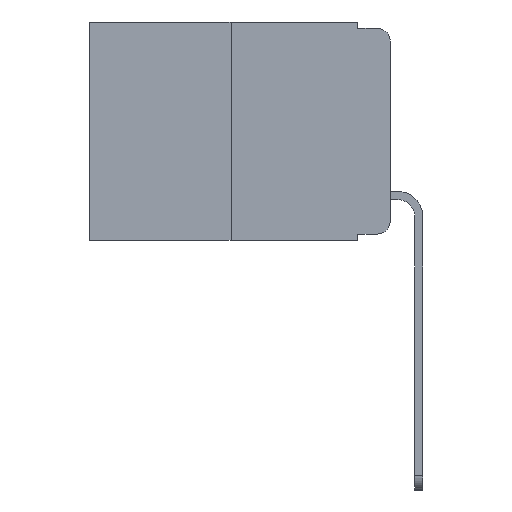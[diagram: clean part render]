
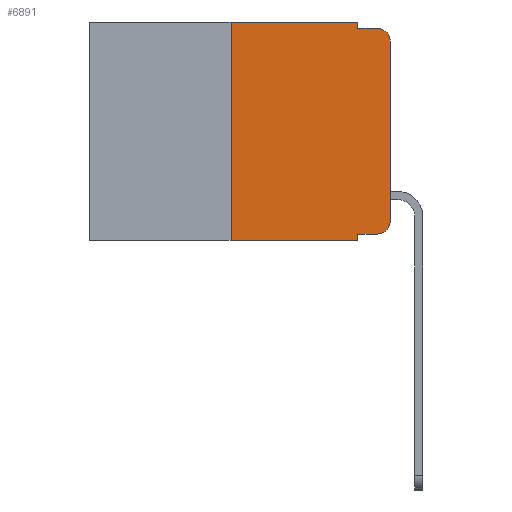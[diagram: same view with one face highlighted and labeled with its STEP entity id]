
A CAD part, left-side view. The second image highlights one B-rep face of the part: STEP entity #6891.
In plain terms, the highlighted planar face has unit normal (-1, 0, 0).
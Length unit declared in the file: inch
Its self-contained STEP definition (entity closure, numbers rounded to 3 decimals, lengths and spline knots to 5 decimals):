
#18 = ORIENTED_EDGE ( 'NONE', *, *, #57, .F. ) ;
#43 = CARTESIAN_POINT ( 'NONE',  ( 0., 0., 0. ) ) ;
#57 = EDGE_CURVE ( 'NONE', #5932, #10891, #1332, .T. ) ;
#103 = VERTEX_POINT ( 'NONE', #6061 ) ;
#205 = AXIS2_PLACEMENT_3D ( 'NONE', #3774, #10359, #4738 ) ;
#323 = ORIENTED_EDGE ( 'NONE', *, *, #4241, .F. ) ;
#609 = CARTESIAN_POINT ( 'NONE',  ( 0., 0.02, -0.333 ) ) ;
#680 = DIRECTION ( 'NONE',  ( 1., 0., 0. ) ) ;
#1033 = ORIENTED_EDGE ( 'NONE', *, *, #2720, .F. ) ;
#1242 = CARTESIAN_POINT ( 'NONE',  ( 0., 0.25, 0. ) ) ;
#1308 = ORIENTED_EDGE ( 'NONE', *, *, #7419, .T. ) ;
#1332 = LINE ( 'NONE', #3484, #6007 ) ;
#1449 = DIRECTION ( 'NONE',  ( 0., -1., 0. ) ) ;
#1610 = CARTESIAN_POINT ( 'NONE',  ( 0., 0., -0.03 ) ) ;
#1893 = ORIENTED_EDGE ( 'NONE', *, *, #2748, .T. ) ;
#1938 = DIRECTION ( 'NONE',  ( 0., -1., 0. ) ) ;
#2084 = DIRECTION ( 'NONE',  ( 0., 0., -1. ) ) ;
#2150 = ORIENTED_EDGE ( 'NONE', *, *, #2764, .F. ) ;
#2442 = VERTEX_POINT ( 'NONE', #1610 ) ;
#2446 = CARTESIAN_POINT ( 'NONE',  ( 0., 0.473, -0.343 ) ) ;
#2636 = ORIENTED_EDGE ( 'NONE', *, *, #9482, .T. ) ;
#2720 = EDGE_CURVE ( 'NONE', #10809, #6787, #6784, .T. ) ;
#2748 = EDGE_CURVE ( 'NONE', #2442, #6787, #11028, .T. ) ;
#2764 = EDGE_CURVE ( 'NONE', #10671, #10809, #3883, .T. ) ;
#2803 = EDGE_CURVE ( 'NONE', #3723, #2442, #7843, .T. ) ;
#3084 = CIRCLE ( 'NONE', #205, 0.02 ) ;
#3091 = CARTESIAN_POINT ( 'NONE',  ( 0., 0.051, 0. ) ) ;
#3484 = CARTESIAN_POINT ( 'NONE',  ( 0., 0.25, 0. ) ) ;
#3723 = VERTEX_POINT ( 'NONE', #11945 ) ;
#3735 = ORIENTED_EDGE ( 'NONE', *, *, #8161, .F. ) ;
#3774 = CARTESIAN_POINT ( 'NONE',  ( 0., 0.02, -0.313 ) ) ;
#3883 = LINE ( 'NONE', #3091, #6157 ) ;
#4241 = EDGE_CURVE ( 'NONE', #10979, #103, #8240, .T. ) ;
#4738 = DIRECTION ( 'NONE',  ( 0., 0., -1. ) ) ;
#4887 = CARTESIAN_POINT ( 'NONE',  ( 0., 0.473, 0. ) ) ;
#5195 = FACE_OUTER_BOUND ( 'NONE', #5410, .T. ) ;
#5410 = EDGE_LOOP ( 'NONE', ( #10068, #1893, #1033, #2150, #3735, #18, #2636, #323, #1308, #9926 ) ) ;
#5591 = VECTOR ( 'NONE', #1449, 39.37008 ) ;
#5630 = VECTOR ( 'NONE', #7836, 39.37008 ) ;
#5920 = LINE ( 'NONE', #2446, #5591 ) ;
#5932 = VERTEX_POINT ( 'NONE', #8410 ) ;
#5979 = DIRECTION ( 'NONE',  ( 0., 0., -1. ) ) ;
#6007 = VECTOR ( 'NONE', #7228, 39.37008 ) ;
#6061 = CARTESIAN_POINT ( 'NONE',  ( 0., 0.051, -0.343 ) ) ;
#6157 = VECTOR ( 'NONE', #2084, 39.37008 ) ;
#6293 = CARTESIAN_POINT ( 'NONE',  ( 0., 0.051, -0.333 ) ) ;
#6436 = LINE ( 'NONE', #10551, #11000 ) ;
#6784 = LINE ( 'NONE', #7641, #8996 ) ;
#6787 = VERTEX_POINT ( 'NONE', #9212 ) ;
#6821 = DIRECTION ( 'NONE',  ( 0., -1., 0. ) ) ;
#6888 = VECTOR ( 'NONE', #1938, 39.37008 ) ;
#6891 = ADVANCED_FACE ( 'NONE', ( #5195 ), #9555, .F. ) ;
#7151 = DIRECTION ( 'NONE',  ( 0., 0., 1. ) ) ;
#7228 = DIRECTION ( 'NONE',  ( 0., 0., 1. ) ) ;
#7317 = EDGE_CURVE ( 'NONE', #10431, #3723, #3084, .T. ) ;
#7419 = EDGE_CURVE ( 'NONE', #10979, #10431, #6436, .T. ) ;
#7641 = CARTESIAN_POINT ( 'NONE',  ( 0., 0.051, -0.01 ) ) ;
#7836 = DIRECTION ( 'NONE',  ( 0., 0., -1. ) ) ;
#7843 = LINE ( 'NONE', #43, #8126 ) ;
#8126 = VECTOR ( 'NONE', #7151, 39.37008 ) ;
#8161 = EDGE_CURVE ( 'NONE', #10891, #10671, #9364, .T. ) ;
#8240 = LINE ( 'NONE', #10496, #5630 ) ;
#8410 = CARTESIAN_POINT ( 'NONE',  ( 0., 0.25, -0.343 ) ) ;
#8667 = CARTESIAN_POINT ( 'NONE',  ( 0., 0.473, 0. ) ) ;
#8963 = CARTESIAN_POINT ( 'NONE',  ( 0., 0.051, -0.01 ) ) ;
#8996 = VECTOR ( 'NONE', #6821, 39.37008 ) ;
#9212 = CARTESIAN_POINT ( 'NONE',  ( 0., 0.02, -0.01 ) ) ;
#9364 = LINE ( 'NONE', #4887, #6888 ) ;
#9482 = EDGE_CURVE ( 'NONE', #5932, #103, #5920, .T. ) ;
#9555 = PLANE ( 'NONE',  #11297 ) ;
#9667 = DIRECTION ( 'NONE',  ( 0., -1., 0. ) ) ;
#9926 = ORIENTED_EDGE ( 'NONE', *, *, #7317, .T. ) ;
#10068 = ORIENTED_EDGE ( 'NONE', *, *, #2803, .T. ) ;
#10359 = DIRECTION ( 'NONE',  ( -1., 0., 0. ) ) ;
#10431 = VERTEX_POINT ( 'NONE', #609 ) ;
#10437 = DIRECTION ( 'NONE',  ( 0., 0., -1. ) ) ;
#10496 = CARTESIAN_POINT ( 'NONE',  ( 0., 0.051, 0. ) ) ;
#10551 = CARTESIAN_POINT ( 'NONE',  ( 0., 0.051, -0.333 ) ) ;
#10671 = VERTEX_POINT ( 'NONE', #11441 ) ;
#10809 = VERTEX_POINT ( 'NONE', #8963 ) ;
#10891 = VERTEX_POINT ( 'NONE', #1242 ) ;
#10979 = VERTEX_POINT ( 'NONE', #6293 ) ;
#11000 = VECTOR ( 'NONE', #9667, 39.37008 ) ;
#11028 = CIRCLE ( 'NONE', #11181, 0.02 ) ;
#11181 = AXIS2_PLACEMENT_3D ( 'NONE', #11844, #11464, #5979 ) ;
#11297 = AXIS2_PLACEMENT_3D ( 'NONE', #8667, #680, #10437 ) ;
#11441 = CARTESIAN_POINT ( 'NONE',  ( 0., 0.051, 0. ) ) ;
#11464 = DIRECTION ( 'NONE',  ( -1., 0., 0. ) ) ;
#11844 = CARTESIAN_POINT ( 'NONE',  ( 0., 0.02, -0.03 ) ) ;
#11945 = CARTESIAN_POINT ( 'NONE',  ( 0., 0., -0.313 ) ) ;
